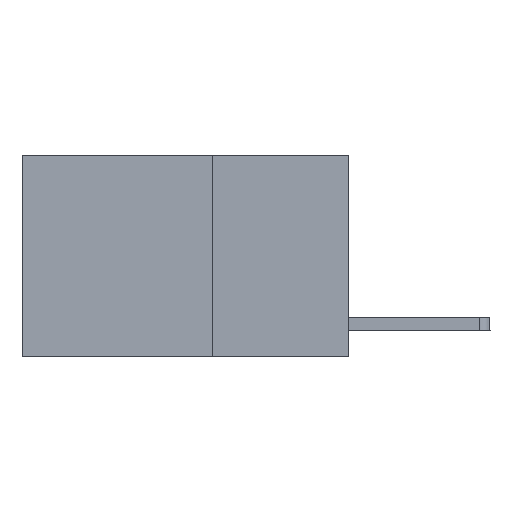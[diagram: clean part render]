
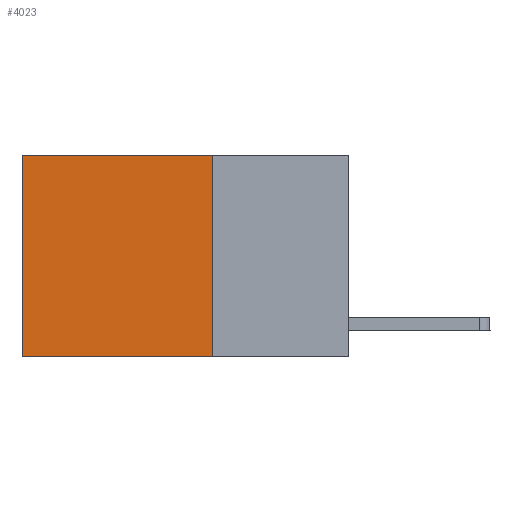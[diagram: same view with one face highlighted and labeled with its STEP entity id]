
A CAD part, left-side view. The second image highlights one B-rep face of the part: STEP entity #4023.
In plain terms, the highlighted planar face has unit normal (-1, 0, 0).
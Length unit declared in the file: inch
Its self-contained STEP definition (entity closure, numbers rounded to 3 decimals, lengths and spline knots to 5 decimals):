
#33 = LINE ( 'NONE', #8532, #4851 ) ;
#50 = ORIENTED_EDGE ( 'NONE', *, *, #9357, .T. ) ;
#132 = DIRECTION ( 'NONE',  ( 0., 0., -1. ) ) ;
#1067 = CARTESIAN_POINT ( 'NONE',  ( 0.2625, 0.25, 0. ) ) ;
#1079 = CARTESIAN_POINT ( 'NONE',  ( 0.2625, 0.25, 0. ) ) ;
#1506 = LINE ( 'NONE', #3943, #4287 ) ;
#1980 = LINE ( 'NONE', #1067, #3818 ) ;
#2062 = EDGE_LOOP ( 'NONE', ( #50, #9960, #7867, #4030 ) ) ;
#2182 = VERTEX_POINT ( 'NONE', #3922 ) ;
#2269 = EDGE_CURVE ( 'NONE', #2182, #10310, #2915, .T. ) ;
#2915 = LINE ( 'NONE', #9815, #7308 ) ;
#3442 = FACE_OUTER_BOUND ( 'NONE', #2062, .T. ) ;
#3496 = DIRECTION ( 'NONE',  ( 1., 0., 0. ) ) ;
#3818 = VECTOR ( 'NONE', #8754, 39.37008 ) ;
#3922 = CARTESIAN_POINT ( 'NONE',  ( 0.2625, 0.25, -0.37 ) ) ;
#3943 = CARTESIAN_POINT ( 'NONE',  ( 0.2625, 0.25, 0. ) ) ;
#4023 = ADVANCED_FACE ( 'NONE', ( #3442 ), #9477, .F. ) ;
#4030 = ORIENTED_EDGE ( 'NONE', *, *, #9941, .T. ) ;
#4287 = VECTOR ( 'NONE', #6477, 39.37008 ) ;
#4473 = VERTEX_POINT ( 'NONE', #6148 ) ;
#4638 = DIRECTION ( 'NONE',  ( 0., 1., 0. ) ) ;
#4851 = VECTOR ( 'NONE', #10229, 39.37008 ) ;
#5776 = VERTEX_POINT ( 'NONE', #9579 ) ;
#6148 = CARTESIAN_POINT ( 'NONE',  ( 0.2625, 0.6, 0. ) ) ;
#6477 = DIRECTION ( 'NONE',  ( 0., 1., 0. ) ) ;
#7308 = VECTOR ( 'NONE', #4638, 39.37008 ) ;
#7867 = ORIENTED_EDGE ( 'NONE', *, *, #9868, .F. ) ;
#8532 = CARTESIAN_POINT ( 'NONE',  ( 0.2625, 0.6, 0. ) ) ;
#8754 = DIRECTION ( 'NONE',  ( 0., 0., -1. ) ) ;
#9357 = EDGE_CURVE ( 'NONE', #4473, #10310, #33, .T. ) ;
#9477 = PLANE ( 'NONE',  #10201 ) ;
#9579 = CARTESIAN_POINT ( 'NONE',  ( 0.2625, 0.25, 0. ) ) ;
#9705 = CARTESIAN_POINT ( 'NONE',  ( 0.2625, 0.6, -0.37 ) ) ;
#9815 = CARTESIAN_POINT ( 'NONE',  ( 0.2625, 0.25, -0.37 ) ) ;
#9868 = EDGE_CURVE ( 'NONE', #5776, #2182, #1980, .T. ) ;
#9941 = EDGE_CURVE ( 'NONE', #5776, #4473, #1506, .T. ) ;
#9960 = ORIENTED_EDGE ( 'NONE', *, *, #2269, .F. ) ;
#10201 = AXIS2_PLACEMENT_3D ( 'NONE', #1079, #3496, #132 ) ;
#10229 = DIRECTION ( 'NONE',  ( 0., 0., -1. ) ) ;
#10310 = VERTEX_POINT ( 'NONE', #9705 ) ;
